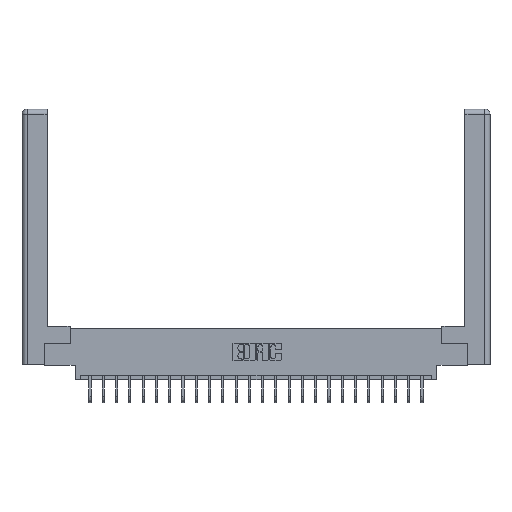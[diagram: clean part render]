
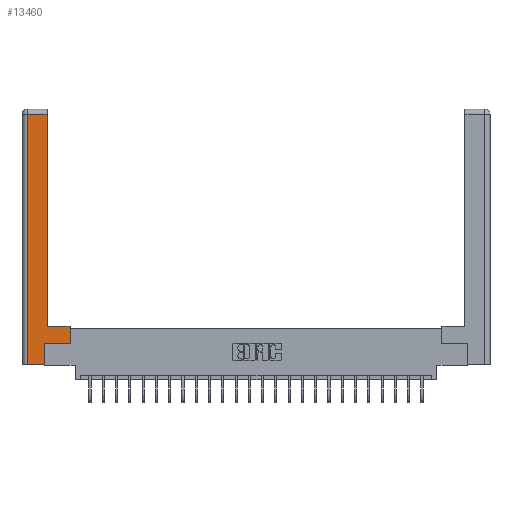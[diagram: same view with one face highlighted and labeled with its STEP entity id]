
A CAD part, top view. The second image highlights one B-rep face of the part: STEP entity #13460.
In plain terms, the highlighted planar face has unit normal (0, 0, 1).
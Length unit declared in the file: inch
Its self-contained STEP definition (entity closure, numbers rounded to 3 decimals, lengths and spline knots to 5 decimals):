
#39 = EDGE_CURVE ( 'NONE', #7747, #11580, #10765, .T. ) ;
#1040 = VERTEX_POINT ( 'NONE', #24226 ) ;
#1114 = LINE ( 'NONE', #9051, #8730 ) ;
#1509 = DIRECTION ( 'NONE',  ( 0., 1., 0. ) ) ;
#2449 = CARTESIAN_POINT ( 'NONE',  ( 0.295, 2.94, 0. ) ) ;
#2668 = ORIENTED_EDGE ( 'NONE', *, *, #2877, .T. ) ;
#2842 = ORIENTED_EDGE ( 'NONE', *, *, #8774, .T. ) ;
#2877 = EDGE_CURVE ( 'NONE', #3352, #20459, #1114, .T. ) ;
#2961 = CARTESIAN_POINT ( 'NONE',  ( 0.295, 0.45, 0. ) ) ;
#3120 = CARTESIAN_POINT ( 'NONE',  ( 0.565, 0.245, 0. ) ) ;
#3352 = VERTEX_POINT ( 'NONE', #3120 ) ;
#3428 = PLANE ( 'NONE',  #8166 ) ;
#4765 = LINE ( 'NONE', #15490, #19074 ) ;
#5190 = CARTESIAN_POINT ( 'NONE',  ( 0.295, 3., 0. ) ) ;
#5910 = DIRECTION ( 'NONE',  ( -1., 0., 0. ) ) ;
#7455 = VERTEX_POINT ( 'NONE', #2961 ) ;
#7526 = LINE ( 'NONE', #14918, #7820 ) ;
#7629 = LINE ( 'NONE', #20782, #10596 ) ;
#7747 = VERTEX_POINT ( 'NONE', #10732 ) ;
#7820 = VECTOR ( 'NONE', #16550, 39.37008 ) ;
#8166 = AXIS2_PLACEMENT_3D ( 'NONE', #8826, #24021, #20011 ) ;
#8167 = VERTEX_POINT ( 'NONE', #2449 ) ;
#8626 = ORIENTED_EDGE ( 'NONE', *, *, #39, .T. ) ;
#8729 = DIRECTION ( 'NONE',  ( 0., 1., 0. ) ) ;
#8730 = VECTOR ( 'NONE', #10791, 39.37008 ) ;
#8774 = EDGE_CURVE ( 'NONE', #11769, #7747, #4765, .T. ) ;
#8801 = CARTESIAN_POINT ( 'NONE',  ( 0.265, 0.245, 0. ) ) ;
#8826 = CARTESIAN_POINT ( 'NONE',  ( 0., 0., 0. ) ) ;
#8989 = VECTOR ( 'NONE', #8729, 39.37008 ) ;
#9051 = CARTESIAN_POINT ( 'NONE',  ( 0.565, 0.45, 0. ) ) ;
#9543 = CARTESIAN_POINT ( 'NONE',  ( 0.0615, 0., 0. ) ) ;
#9775 = ORIENTED_EDGE ( 'NONE', *, *, #14181, .T. ) ;
#9933 = ORIENTED_EDGE ( 'NONE', *, *, #17326, .T. ) ;
#10596 = VECTOR ( 'NONE', #5910, 39.37008 ) ;
#10732 = CARTESIAN_POINT ( 'NONE',  ( 0.265, 0., 0. ) ) ;
#10765 = LINE ( 'NONE', #8801, #8989 ) ;
#10791 = DIRECTION ( 'NONE',  ( 0., 1., 0. ) ) ;
#11041 = CARTESIAN_POINT ( 'NONE',  ( 0.0615, 0., 0. ) ) ;
#11122 = DIRECTION ( 'NONE',  ( 0., -1., 0. ) ) ;
#11580 = VERTEX_POINT ( 'NONE', #14384 ) ;
#11769 = VERTEX_POINT ( 'NONE', #9543 ) ;
#11772 = EDGE_CURVE ( 'NONE', #20459, #7455, #7629, .T. ) ;
#13460 = ADVANCED_FACE ( 'NONE', ( #15165 ), #3428, .F. ) ;
#13876 = ORIENTED_EDGE ( 'NONE', *, *, #11772, .T. ) ;
#13878 = VECTOR ( 'NONE', #11122, 39.37008 ) ;
#14145 = EDGE_CURVE ( 'NONE', #7455, #8167, #15428, .T. ) ;
#14181 = EDGE_CURVE ( 'NONE', #11580, #3352, #7526, .T. ) ;
#14384 = CARTESIAN_POINT ( 'NONE',  ( 0.265, 0.245, 0. ) ) ;
#14890 = EDGE_CURVE ( 'NONE', #8167, #1040, #19787, .T. ) ;
#14918 = CARTESIAN_POINT ( 'NONE',  ( 0.565, 0.245, 0. ) ) ;
#15165 = FACE_OUTER_BOUND ( 'NONE', #20164, .T. ) ;
#15428 = LINE ( 'NONE', #5190, #22459 ) ;
#15490 = CARTESIAN_POINT ( 'NONE',  ( 0.265, 0., 0. ) ) ;
#16478 = LINE ( 'NONE', #11041, #13878 ) ;
#16550 = DIRECTION ( 'NONE',  ( 1., 0., 0. ) ) ;
#17326 = EDGE_CURVE ( 'NONE', #1040, #11769, #16478, .T. ) ;
#18563 = ORIENTED_EDGE ( 'NONE', *, *, #14890, .T. ) ;
#19074 = VECTOR ( 'NONE', #21211, 39.37008 ) ;
#19787 = LINE ( 'NONE', #21557, #23575 ) ;
#19856 = CARTESIAN_POINT ( 'NONE',  ( 0.565, 0.45, 0. ) ) ;
#20011 = DIRECTION ( 'NONE',  ( -1., 0., 0. ) ) ;
#20164 = EDGE_LOOP ( 'NONE', ( #21082, #18563, #9933, #2842, #8626, #9775, #2668, #13876 ) ) ;
#20459 = VERTEX_POINT ( 'NONE', #19856 ) ;
#20782 = CARTESIAN_POINT ( 'NONE',  ( 0.295, 0.45, 0. ) ) ;
#21082 = ORIENTED_EDGE ( 'NONE', *, *, #14145, .T. ) ;
#21211 = DIRECTION ( 'NONE',  ( 1., 0., 0. ) ) ;
#21557 = CARTESIAN_POINT ( 'NONE',  ( 0.0615, 2.94, 0. ) ) ;
#22459 = VECTOR ( 'NONE', #1509, 39.37008 ) ;
#23438 = DIRECTION ( 'NONE',  ( -1., 0., 0. ) ) ;
#23575 = VECTOR ( 'NONE', #23438, 39.37008 ) ;
#24021 = DIRECTION ( 'NONE',  ( 0., 0., -1. ) ) ;
#24226 = CARTESIAN_POINT ( 'NONE',  ( 0.0615, 2.94, 0. ) ) ;
